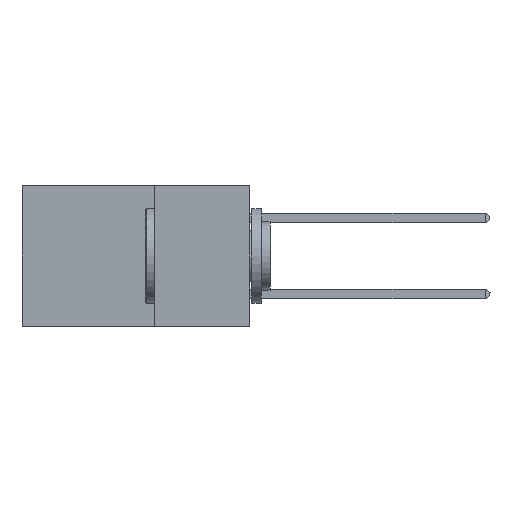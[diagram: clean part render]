
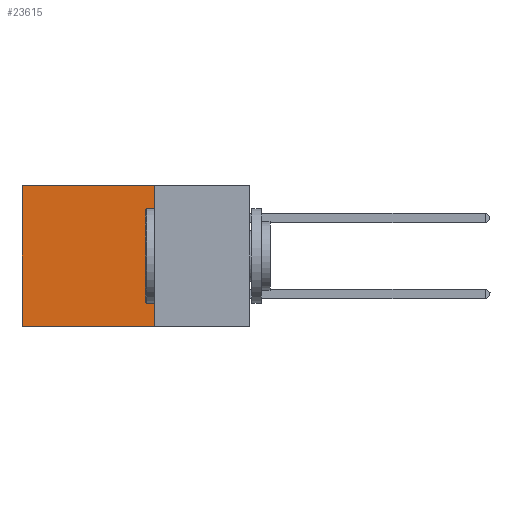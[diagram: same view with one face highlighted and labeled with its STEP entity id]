
A CAD part, left-side view. The second image highlights one B-rep face of the part: STEP entity #23615.
In plain terms, the highlighted planar face has unit normal (-1, 0, 0).
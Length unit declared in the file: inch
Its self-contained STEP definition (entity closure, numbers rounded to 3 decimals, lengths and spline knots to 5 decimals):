
#1194 = VERTEX_POINT ( 'NONE', #12875 ) ;
#1810 = VECTOR ( 'NONE', #21912, 39.37008 ) ;
#2021 = CARTESIAN_POINT ( 'NONE',  ( 0.2875, 0.25, 0. ) ) ;
#2768 = VERTEX_POINT ( 'NONE', #7300 ) ;
#2918 = PLANE ( 'NONE',  #16860 ) ;
#4944 = EDGE_CURVE ( 'NONE', #2768, #12671, #23856, .T. ) ;
#5502 = CARTESIAN_POINT ( 'NONE',  ( 0.2875, 0.25, -0.37 ) ) ;
#5554 = FACE_OUTER_BOUND ( 'NONE', #23350, .T. ) ;
#5803 = ORIENTED_EDGE ( 'NONE', *, *, #13411, .F. ) ;
#7039 = LINE ( 'NONE', #19995, #1810 ) ;
#7300 = CARTESIAN_POINT ( 'NONE',  ( 0.2875, 0.25, 0. ) ) ;
#8073 = VECTOR ( 'NONE', #16134, 39.37008 ) ;
#9690 = DIRECTION ( 'NONE',  ( 0., 0., -1. ) ) ;
#10045 = VERTEX_POINT ( 'NONE', #17727 ) ;
#10612 = VECTOR ( 'NONE', #9690, 39.37008 ) ;
#12047 = DIRECTION ( 'NONE',  ( 0., 1., 0. ) ) ;
#12667 = EDGE_CURVE ( 'NONE', #10045, #1194, #7039, .T. ) ;
#12671 = VERTEX_POINT ( 'NONE', #5502 ) ;
#12875 = CARTESIAN_POINT ( 'NONE',  ( 0.2875, 0.6, -0.37 ) ) ;
#12987 = LINE ( 'NONE', #19714, #8073 ) ;
#13411 = EDGE_CURVE ( 'NONE', #12671, #1194, #12987, .T. ) ;
#13597 = ORIENTED_EDGE ( 'NONE', *, *, #12667, .T. ) ;
#15737 = DIRECTION ( 'NONE',  ( 0., 0., -1. ) ) ;
#15780 = LINE ( 'NONE', #19536, #22922 ) ;
#16134 = DIRECTION ( 'NONE',  ( 0., 1., 0. ) ) ;
#16827 = ORIENTED_EDGE ( 'NONE', *, *, #4944, .F. ) ;
#16860 = AXIS2_PLACEMENT_3D ( 'NONE', #21157, #23001, #15737 ) ;
#17727 = CARTESIAN_POINT ( 'NONE',  ( 0.2875, 0.6, 0. ) ) ;
#19536 = CARTESIAN_POINT ( 'NONE',  ( 0.2875, 0.25, 0. ) ) ;
#19714 = CARTESIAN_POINT ( 'NONE',  ( 0.2875, 0.25, -0.37 ) ) ;
#19995 = CARTESIAN_POINT ( 'NONE',  ( 0.2875, 0.6, 0. ) ) ;
#20521 = EDGE_CURVE ( 'NONE', #2768, #10045, #15780, .T. ) ;
#20924 = ORIENTED_EDGE ( 'NONE', *, *, #20521, .T. ) ;
#21157 = CARTESIAN_POINT ( 'NONE',  ( 0.2875, 0.25, 0. ) ) ;
#21912 = DIRECTION ( 'NONE',  ( 0., 0., -1. ) ) ;
#22922 = VECTOR ( 'NONE', #12047, 39.37008 ) ;
#23001 = DIRECTION ( 'NONE',  ( 1., 0., 0. ) ) ;
#23350 = EDGE_LOOP ( 'NONE', ( #13597, #5803, #16827, #20924 ) ) ;
#23615 = ADVANCED_FACE ( 'NONE', ( #5554 ), #2918, .F. ) ;
#23856 = LINE ( 'NONE', #2021, #10612 ) ;
